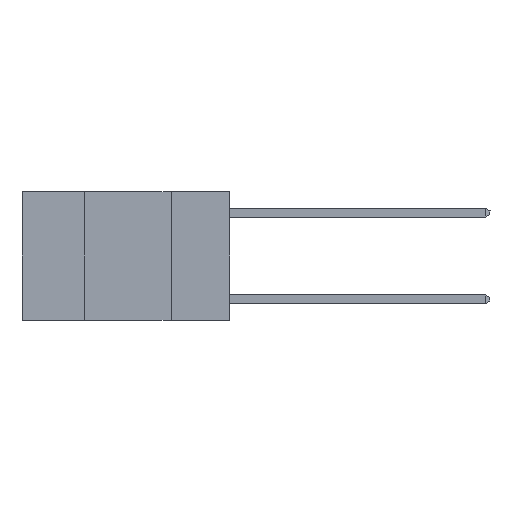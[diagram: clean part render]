
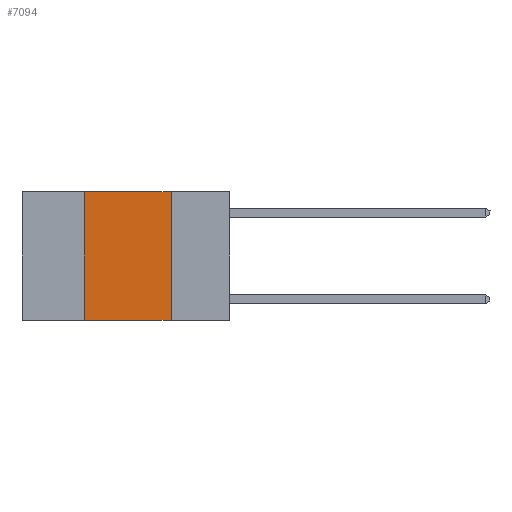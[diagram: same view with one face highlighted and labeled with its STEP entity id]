
A CAD part, left-side view. The second image highlights one B-rep face of the part: STEP entity #7094.
In plain terms, the highlighted planar face has unit normal (-1, 0, 0).
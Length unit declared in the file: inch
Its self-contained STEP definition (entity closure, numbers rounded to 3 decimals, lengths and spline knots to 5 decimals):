
#1008 = EDGE_CURVE ( 'NONE', #14121, #11418, #10388, .T. ) ;
#1020 = CARTESIAN_POINT ( 'NONE',  ( 0., 0.17, 0. ) ) ;
#1720 = EDGE_CURVE ( 'NONE', #11418, #6396, #14978, .T. ) ;
#1776 = FACE_OUTER_BOUND ( 'NONE', #4974, .T. ) ;
#1855 = LINE ( 'NONE', #14425, #10257 ) ;
#2324 = DIRECTION ( 'NONE',  ( 0., 0., -1. ) ) ;
#2684 = VECTOR ( 'NONE', #9009, 39.37008 ) ;
#3196 = DIRECTION ( 'NONE',  ( 0., -1., 0. ) ) ;
#3198 = ORIENTED_EDGE ( 'NONE', *, *, #1720, .F. ) ;
#3221 = EDGE_CURVE ( 'NONE', #18074, #14121, #1855, .T. ) ;
#3334 = DIRECTION ( 'NONE',  ( 0., 0., 1. ) ) ;
#4489 = LINE ( 'NONE', #10131, #7990 ) ;
#4569 = CARTESIAN_POINT ( 'NONE',  ( 0., 0.42, 0. ) ) ;
#4974 = EDGE_LOOP ( 'NONE', ( #3198, #5760, #14290, #5302 ) ) ;
#5302 = ORIENTED_EDGE ( 'NONE', *, *, #11011, .T. ) ;
#5760 = ORIENTED_EDGE ( 'NONE', *, *, #1008, .F. ) ;
#6396 = VERTEX_POINT ( 'NONE', #13722 ) ;
#7003 = AXIS2_PLACEMENT_3D ( 'NONE', #7425, #13065, #8531 ) ;
#7094 = ADVANCED_FACE ( 'NONE', ( #1776 ), #17295, .F. ) ;
#7425 = CARTESIAN_POINT ( 'NONE',  ( 0., 0.6, 0. ) ) ;
#7990 = VECTOR ( 'NONE', #3196, 39.37008 ) ;
#8531 = DIRECTION ( 'NONE',  ( 0., 0., -1. ) ) ;
#8975 = CARTESIAN_POINT ( 'NONE',  ( 0., 0.17, 0. ) ) ;
#9009 = DIRECTION ( 'NONE',  ( 0., -1., 0. ) ) ;
#10131 = CARTESIAN_POINT ( 'NONE',  ( 0., 0.6, -0.37 ) ) ;
#10257 = VECTOR ( 'NONE', #3334, 39.37008 ) ;
#10388 = LINE ( 'NONE', #17411, #2684 ) ;
#11011 = EDGE_CURVE ( 'NONE', #18074, #6396, #4489, .T. ) ;
#11418 = VERTEX_POINT ( 'NONE', #8975 ) ;
#13065 = DIRECTION ( 'NONE',  ( 1., 0., 0. ) ) ;
#13722 = CARTESIAN_POINT ( 'NONE',  ( 0., 0.17, -0.37 ) ) ;
#13932 = CARTESIAN_POINT ( 'NONE',  ( 0., 0.42, -0.37 ) ) ;
#14121 = VERTEX_POINT ( 'NONE', #4569 ) ;
#14192 = VECTOR ( 'NONE', #2324, 39.37008 ) ;
#14290 = ORIENTED_EDGE ( 'NONE', *, *, #3221, .F. ) ;
#14425 = CARTESIAN_POINT ( 'NONE',  ( 0., 0.42, 0. ) ) ;
#14978 = LINE ( 'NONE', #1020, #14192 ) ;
#17295 = PLANE ( 'NONE',  #7003 ) ;
#17411 = CARTESIAN_POINT ( 'NONE',  ( 0., 0.6, 0. ) ) ;
#18074 = VERTEX_POINT ( 'NONE', #13932 ) ;
